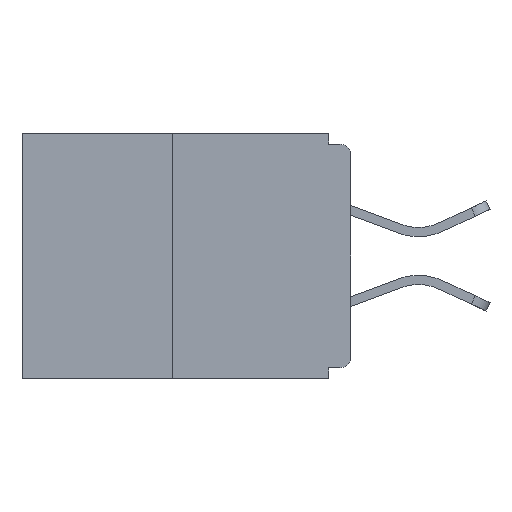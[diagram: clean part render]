
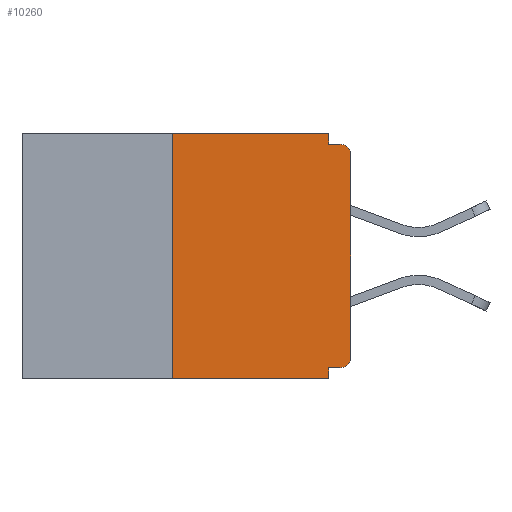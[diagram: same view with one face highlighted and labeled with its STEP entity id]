
A CAD part, left-side view. The second image highlights one B-rep face of the part: STEP entity #10260.
In plain terms, the highlighted planar face has unit normal (-1, 0, 0).
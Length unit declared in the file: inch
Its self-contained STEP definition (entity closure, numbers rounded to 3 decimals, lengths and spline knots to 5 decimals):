
#33 = CARTESIAN_POINT ( 'NONE',  ( 0., 0.031, 0. ) ) ;
#106 = ORIENTED_EDGE ( 'NONE', *, *, #3509, .T. ) ;
#227 = DIRECTION ( 'NONE',  ( 0., 0., -1. ) ) ;
#441 = DIRECTION ( 'NONE',  ( 0., 0., -1. ) ) ;
#444 = CARTESIAN_POINT ( 'NONE',  ( 0., 0.031, -0.015 ) ) ;
#487 = EDGE_LOOP ( 'NONE', ( #2677, #5813, #10942, #1559, #13926, #6838, #106, #9073, #13552, #12066 ) ) ;
#562 = AXIS2_PLACEMENT_3D ( 'NONE', #2686, #6339, #227 ) ;
#604 = CARTESIAN_POINT ( 'NONE',  ( 0., 0., 0. ) ) ;
#711 = CARTESIAN_POINT ( 'NONE',  ( 0., 0., -0.328 ) ) ;
#838 = EDGE_CURVE ( 'NONE', #7902, #7835, #7564, .T. ) ;
#1299 = EDGE_CURVE ( 'NONE', #12605, #1543, #8701, .T. ) ;
#1543 = VERTEX_POINT ( 'NONE', #444 ) ;
#1559 = ORIENTED_EDGE ( 'NONE', *, *, #8782, .F. ) ;
#1694 = CIRCLE ( 'NONE', #11677, 0.015 ) ;
#2210 = DIRECTION ( 'NONE',  ( 0., 0., -1. ) ) ;
#2262 = CARTESIAN_POINT ( 'NONE',  ( 0., 0., -0.015 ) ) ;
#2375 = CARTESIAN_POINT ( 'NONE',  ( 0., 0.25, 0. ) ) ;
#2549 = VECTOR ( 'NONE', #11753, 39.37008 ) ;
#2610 = LINE ( 'NONE', #2375, #3924 ) ;
#2677 = ORIENTED_EDGE ( 'NONE', *, *, #7731, .F. ) ;
#2686 = CARTESIAN_POINT ( 'NONE',  ( 0., 0.015, -0.313 ) ) ;
#2858 = DIRECTION ( 'NONE',  ( 1., 0., 0. ) ) ;
#3294 = VECTOR ( 'NONE', #12370, 39.37008 ) ;
#3340 = CARTESIAN_POINT ( 'NONE',  ( 0., 0.031, 0. ) ) ;
#3351 = EDGE_CURVE ( 'NONE', #4467, #12179, #1694, .T. ) ;
#3509 = EDGE_CURVE ( 'NONE', #8556, #4467, #8624, .T. ) ;
#3924 = VECTOR ( 'NONE', #12131, 39.37008 ) ;
#4467 = VERTEX_POINT ( 'NONE', #11273 ) ;
#4789 = FACE_OUTER_BOUND ( 'NONE', #487, .T. ) ;
#5226 = EDGE_CURVE ( 'NONE', #9305, #13547, #2610, .T. ) ;
#5813 = ORIENTED_EDGE ( 'NONE', *, *, #5226, .F. ) ;
#5869 = DIRECTION ( 'NONE',  ( 0., 0., -1. ) ) ;
#6118 = LINE ( 'NONE', #14860, #9587 ) ;
#6339 = DIRECTION ( 'NONE',  ( -1., 0., 0. ) ) ;
#6461 = CARTESIAN_POINT ( 'NONE',  ( 0., 0.46, 0. ) ) ;
#6483 = CARTESIAN_POINT ( 'NONE',  ( 0., 0., -0.313 ) ) ;
#6838 = ORIENTED_EDGE ( 'NONE', *, *, #12294, .T. ) ;
#7328 = VECTOR ( 'NONE', #15807, 39.37008 ) ;
#7564 = LINE ( 'NONE', #711, #2549 ) ;
#7621 = CARTESIAN_POINT ( 'NONE',  ( 0., 0.015, -0.015 ) ) ;
#7622 = DIRECTION ( 'NONE',  ( 0., -1., 0. ) ) ;
#7664 = CARTESIAN_POINT ( 'NONE',  ( 0., 0.015, -0.328 ) ) ;
#7731 = EDGE_CURVE ( 'NONE', #13547, #12605, #8131, .T. ) ;
#7835 = VERTEX_POINT ( 'NONE', #11158 ) ;
#7902 = VERTEX_POINT ( 'NONE', #7664 ) ;
#8131 = LINE ( 'NONE', #14899, #3294 ) ;
#8231 = EDGE_CURVE ( 'NONE', #1543, #12179, #10018, .T. ) ;
#8556 = VERTEX_POINT ( 'NONE', #6483 ) ;
#8624 = LINE ( 'NONE', #604, #11485 ) ;
#8675 = CIRCLE ( 'NONE', #562, 0.015 ) ;
#8701 = LINE ( 'NONE', #3340, #14245 ) ;
#8782 = EDGE_CURVE ( 'NONE', #7835, #9040, #11909, .T. ) ;
#9039 = VECTOR ( 'NONE', #5869, 39.37008 ) ;
#9040 = VERTEX_POINT ( 'NONE', #11318 ) ;
#9073 = ORIENTED_EDGE ( 'NONE', *, *, #3351, .T. ) ;
#9305 = VERTEX_POINT ( 'NONE', #14290 ) ;
#9480 = CARTESIAN_POINT ( 'NONE',  ( 0., 0.031, -0.343 ) ) ;
#9587 = VECTOR ( 'NONE', #7622, 39.37008 ) ;
#10018 = LINE ( 'NONE', #2262, #7328 ) ;
#10059 = PLANE ( 'NONE',  #15352 ) ;
#10125 = CARTESIAN_POINT ( 'NONE',  ( 0., 0.25, 0. ) ) ;
#10186 = EDGE_CURVE ( 'NONE', #9305, #9040, #6118, .T. ) ;
#10260 = ADVANCED_FACE ( 'NONE', ( #4789 ), #10059, .F. ) ;
#10540 = DIRECTION ( 'NONE',  ( 0., 0., 1. ) ) ;
#10942 = ORIENTED_EDGE ( 'NONE', *, *, #10186, .T. ) ;
#11158 = CARTESIAN_POINT ( 'NONE',  ( 0., 0.031, -0.328 ) ) ;
#11273 = CARTESIAN_POINT ( 'NONE',  ( 0., 0., -0.03 ) ) ;
#11318 = CARTESIAN_POINT ( 'NONE',  ( 0., 0.031, -0.343 ) ) ;
#11485 = VECTOR ( 'NONE', #10540, 39.37008 ) ;
#11677 = AXIS2_PLACEMENT_3D ( 'NONE', #15003, #12562, #441 ) ;
#11753 = DIRECTION ( 'NONE',  ( 0., 1., 0. ) ) ;
#11909 = LINE ( 'NONE', #9480, #9039 ) ;
#12066 = ORIENTED_EDGE ( 'NONE', *, *, #1299, .F. ) ;
#12131 = DIRECTION ( 'NONE',  ( 0., 0., 1. ) ) ;
#12179 = VERTEX_POINT ( 'NONE', #7621 ) ;
#12294 = EDGE_CURVE ( 'NONE', #7902, #8556, #8675, .T. ) ;
#12370 = DIRECTION ( 'NONE',  ( 0., -1., 0. ) ) ;
#12562 = DIRECTION ( 'NONE',  ( -1., 0., 0. ) ) ;
#12605 = VERTEX_POINT ( 'NONE', #33 ) ;
#12636 = DIRECTION ( 'NONE',  ( 0., 0., -1. ) ) ;
#13547 = VERTEX_POINT ( 'NONE', #10125 ) ;
#13552 = ORIENTED_EDGE ( 'NONE', *, *, #8231, .F. ) ;
#13926 = ORIENTED_EDGE ( 'NONE', *, *, #838, .F. ) ;
#14245 = VECTOR ( 'NONE', #2210, 39.37008 ) ;
#14290 = CARTESIAN_POINT ( 'NONE',  ( 0., 0.25, -0.343 ) ) ;
#14860 = CARTESIAN_POINT ( 'NONE',  ( 0., 0.46, -0.343 ) ) ;
#14899 = CARTESIAN_POINT ( 'NONE',  ( 0., 0.46, 0. ) ) ;
#15003 = CARTESIAN_POINT ( 'NONE',  ( 0., 0.015, -0.03 ) ) ;
#15352 = AXIS2_PLACEMENT_3D ( 'NONE', #6461, #2858, #12636 ) ;
#15807 = DIRECTION ( 'NONE',  ( 0., -1., 0. ) ) ;
